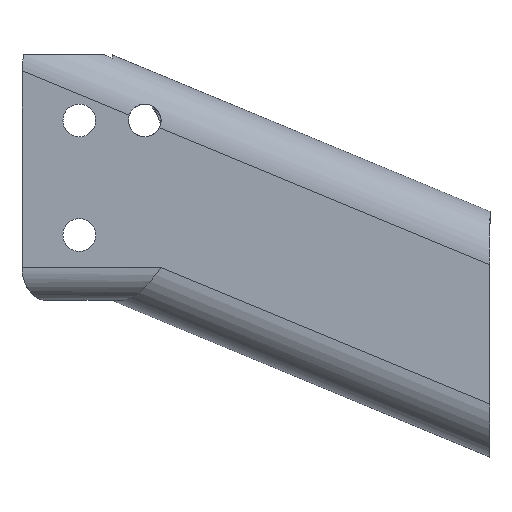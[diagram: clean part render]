
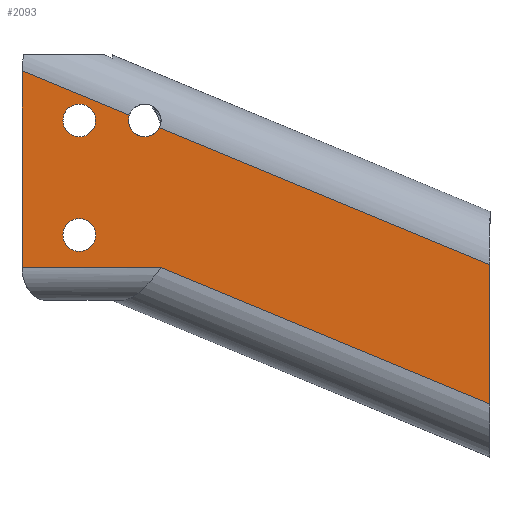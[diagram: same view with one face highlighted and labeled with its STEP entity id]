
A CAD part, left-side view. The second image highlights one B-rep face of the part: STEP entity #2093.
In plain terms, the highlighted planar face has unit normal (-1, 0, 0).
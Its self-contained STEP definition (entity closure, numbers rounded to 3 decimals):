
#119 = CARTESIAN_POINT ( 'NONE',  ( 6.871, -0.974, -9.567 ) ) ;
#329 = CARTESIAN_POINT ( 'NONE',  ( 6.871, 23.594, -61.382 ) ) ;
#330 = DIRECTION ( 'NONE',  ( 0., 0., 1. ) ) ;
#345 = CARTESIAN_POINT ( 'NONE',  ( 6.871, -6.673, -11.928 ) ) ;
#347 = DIRECTION ( 'NONE',  ( 0., 0.924, 0.383 ) ) ;
#348 = CARTESIAN_POINT ( 'NONE',  ( 6.871, -6.673, -11.928 ) ) ;
#354 = DIRECTION ( 'NONE',  ( 0., 0., 1. ) ) ;
#355 = DIRECTION ( 'NONE',  ( -1., 0., 0. ) ) ;
#356 = CARTESIAN_POINT ( 'NONE',  ( 6.871, 10.469, -10.757 ) ) ;
#363 = DIRECTION ( 'NONE',  ( 0., 0.924, 0.383 ) ) ;
#384 = DIRECTION ( 'NONE',  ( 0., 0., 1. ) ) ;
#386 = DIRECTION ( 'NONE',  ( -1., 0., 0. ) ) ;
#387 = CARTESIAN_POINT ( 'NONE',  ( 6.871, 10.469, -37.007 ) ) ;
#404 = CARTESIAN_POINT ( 'NONE',  ( 6.871, -7.887, -12.43 ) ) ;
#414 = CARTESIAN_POINT ( 'NONE',  ( 6.871, -4.531, -14.507 ) ) ;
#445 = DIRECTION ( 'NONE',  ( 0., 0., -1. ) ) ;
#447 = DIRECTION ( 'NONE',  ( 1., 0., 0. ) ) ;
#457 = CARTESIAN_POINT ( 'NONE',  ( 6.871, -7.597, -9.698 ) ) ;
#460 = PLANE ( 'NONE',  #1208 ) ;
#506 = CARTESIAN_POINT ( 'NONE',  ( 6.871, 10.469, -37.007 ) ) ;
#508 = DIRECTION ( 'NONE',  ( -1., 0., 0. ) ) ;
#568 = CARTESIAN_POINT ( 'NONE',  ( 6.871, 10.469, -7.007 ) ) ;
#580 = DIRECTION ( 'NONE',  ( 0., 0., 1. ) ) ;
#582 = DIRECTION ( 'NONE',  ( -1., 0., 0. ) ) ;
#584 = CARTESIAN_POINT ( 'NONE',  ( 6.871, -4.531, -10.757 ) ) ;
#590 = CARTESIAN_POINT ( 'NONE',  ( 6.871, 10.469, -14.507 ) ) ;
#643 = CARTESIAN_POINT ( 'NONE',  ( 6.871, 23.594, 0.609 ) ) ;
#660 = EDGE_CURVE ( 'NONE', #1981, #1991, #1096, .T. ) ;
#666 = LINE ( 'NONE', #897, #675 ) ;
#675 = VECTOR ( 'NONE', #904, 1000. ) ;
#679 = VECTOR ( 'NONE', #1345, 1000. ) ;
#682 = LINE ( 'NONE', #1343, #679 ) ;
#698 = VECTOR ( 'NONE', #330, 1000. ) ;
#700 = VECTOR ( 'NONE', #347, 1000. ) ;
#702 = LINE ( 'NONE', #329, #698 ) ;
#707 = LINE ( 'NONE', #348, #711 ) ;
#709 = LINE ( 'NONE', #345, #700 ) ;
#711 = VECTOR ( 'NONE', #363, 1000. ) ;
#718 = CIRCLE ( 'NONE', #1191, 3.75 ) ;
#739 = CIRCLE ( 'NONE', #1203, 3.75 ) ;
#747 = FACE_BOUND ( 'NONE', #1860, .T. ) ;
#750 = FACE_BOUND ( 'NONE', #1411, .T. ) ;
#757 = FACE_OUTER_BOUND ( 'NONE', #1301, .T. ) ;
#810 = CIRCLE ( 'NONE', #1298, 3.75 ) ;
#877 = LINE ( 'NONE', #1543, #907 ) ;
#897 = CARTESIAN_POINT ( 'NONE',  ( 6.871, -87.95, -77.49 ) ) ;
#904 = DIRECTION ( 'NONE',  ( 0., -0.924, -0.383 ) ) ;
#907 = VECTOR ( 'NONE', #1540, 1000. ) ;
#1012 = CIRCLE ( 'NONE', #1604, 3.75 ) ;
#1036 = CIRCLE ( 'NONE', #1613, 3.75 ) ;
#1037 = EDGE_CURVE ( 'NONE', #2305, #2112, #1036, .T. ) ;
#1096 = CIRCLE ( 'NONE', #1703, 3.75 ) ;
#1099 = DIRECTION ( 'NONE',  ( 0., 0., 1. ) ) ;
#1109 = EDGE_CURVE ( 'NONE', #2047, #2051, #1012, .T. ) ;
#1191 = AXIS2_PLACEMENT_3D ( 'NONE', #356, #355, #354 ) ;
#1203 = AXIS2_PLACEMENT_3D ( 'NONE', #387, #386, #384 ) ;
#1208 = AXIS2_PLACEMENT_3D ( 'NONE', #457, #447, #445 ) ;
#1298 = AXIS2_PLACEMENT_3D ( 'NONE', #584, #582, #580 ) ;
#1301 = EDGE_LOOP ( 'NONE', ( #1615, #1621, #1642, #1653, #1656, #1661, #1665, #1667 ) ) ;
#1343 = CARTESIAN_POINT ( 'NONE',  ( 6.871, -26.428, -44.507 ) ) ;
#1345 = DIRECTION ( 'NONE',  ( 0., -1., 0. ) ) ;
#1395 = VERTEX_POINT ( 'NONE', #2120 ) ;
#1411 = EDGE_LOOP ( 'NONE', ( #1605, #1609 ) ) ;
#1450 = CARTESIAN_POINT ( 'NONE',  ( 6.871, -8.322, -44.507 ) ) ;
#1453 = CARTESIAN_POINT ( 'NONE',  ( 6.871, 10.469, -33.257 ) ) ;
#1477 = CARTESIAN_POINT ( 'NONE',  ( 6.871, 10.469, -40.757 ) ) ;
#1486 = VERTEX_POINT ( 'NONE', #2058 ) ;
#1540 = DIRECTION ( 'NONE',  ( 0., 0., -1. ) ) ;
#1543 = CARTESIAN_POINT ( 'NONE',  ( 6.871, -83.644, -9.698 ) ) ;
#1574 = ORIENTED_EDGE ( 'NONE', *, *, #2123, .F. ) ;
#1576 = ORIENTED_EDGE ( 'NONE', *, *, #660, .F. ) ;
#1604 = AXIS2_PLACEMENT_3D ( 'NONE', #2157, #2150, #2144 ) ;
#1605 = ORIENTED_EDGE ( 'NONE', *, *, #2130, .F. ) ;
#1609 = ORIENTED_EDGE ( 'NONE', *, *, #1109, .F. ) ;
#1613 = AXIS2_PLACEMENT_3D ( 'NONE', #2304, #2301, #2300 ) ;
#1615 = ORIENTED_EDGE ( 'NONE', *, *, #2138, .T. ) ;
#1621 = ORIENTED_EDGE ( 'NONE', *, *, #2038, .F. ) ;
#1642 = ORIENTED_EDGE ( 'NONE', *, *, #1037, .F. ) ;
#1653 = ORIENTED_EDGE ( 'NONE', *, *, #2145, .T. ) ;
#1656 = ORIENTED_EDGE ( 'NONE', *, *, #2158, .F. ) ;
#1661 = ORIENTED_EDGE ( 'NONE', *, *, #2185, .T. ) ;
#1665 = ORIENTED_EDGE ( 'NONE', *, *, #2201, .T. ) ;
#1667 = ORIENTED_EDGE ( 'NONE', *, *, #1962, .F. ) ;
#1703 = AXIS2_PLACEMENT_3D ( 'NONE', #506, #508, #1099 ) ;
#1839 = VERTEX_POINT ( 'NONE', #1920 ) ;
#1860 = EDGE_LOOP ( 'NONE', ( #1574, #1576 ) ) ;
#1920 = CARTESIAN_POINT ( 'NONE',  ( 6.871, -83.644, -43.81 ) ) ;
#1962 = EDGE_CURVE ( 'NONE', #1839, #1486, #877, .T. ) ;
#1981 = VERTEX_POINT ( 'NONE', #1477 ) ;
#1991 = VERTEX_POINT ( 'NONE', #1453 ) ;
#1992 = VERTEX_POINT ( 'NONE', #1450 ) ;
#2038 = EDGE_CURVE ( 'NONE', #2112, #2122, #810, .T. ) ;
#2047 = VERTEX_POINT ( 'NONE', #590 ) ;
#2051 = VERTEX_POINT ( 'NONE', #568 ) ;
#2058 = CARTESIAN_POINT ( 'NONE',  ( 6.871, -83.644, -75.706 ) ) ;
#2093 = ADVANCED_FACE ( 'NONE', ( #747, #750, #757 ), #460, .F. ) ;
#2112 = VERTEX_POINT ( 'NONE', #414 ) ;
#2120 = CARTESIAN_POINT ( 'NONE',  ( 6.871, 23.594, -44.507 ) ) ;
#2122 = VERTEX_POINT ( 'NONE', #404 ) ;
#2123 = EDGE_CURVE ( 'NONE', #1991, #1981, #739, .T. ) ;
#2130 = EDGE_CURVE ( 'NONE', #2051, #2047, #718, .T. ) ;
#2138 = EDGE_CURVE ( 'NONE', #1839, #2122, #707, .T. ) ;
#2144 = DIRECTION ( 'NONE',  ( 0., 0., 1. ) ) ;
#2145 = EDGE_CURVE ( 'NONE', #2305, #2347, #709, .T. ) ;
#2150 = DIRECTION ( 'NONE',  ( -1., 0., 0. ) ) ;
#2157 = CARTESIAN_POINT ( 'NONE',  ( 6.871, 10.469, -10.757 ) ) ;
#2158 = EDGE_CURVE ( 'NONE', #1395, #2347, #702, .T. ) ;
#2185 = EDGE_CURVE ( 'NONE', #1395, #1992, #682, .T. ) ;
#2201 = EDGE_CURVE ( 'NONE', #1992, #1486, #666, .T. ) ;
#2300 = DIRECTION ( 'NONE',  ( 0., 0., 1. ) ) ;
#2301 = DIRECTION ( 'NONE',  ( -1., 0., 0. ) ) ;
#2304 = CARTESIAN_POINT ( 'NONE',  ( 6.871, -4.531, -10.757 ) ) ;
#2305 = VERTEX_POINT ( 'NONE', #119 ) ;
#2347 = VERTEX_POINT ( 'NONE', #643 ) ;
